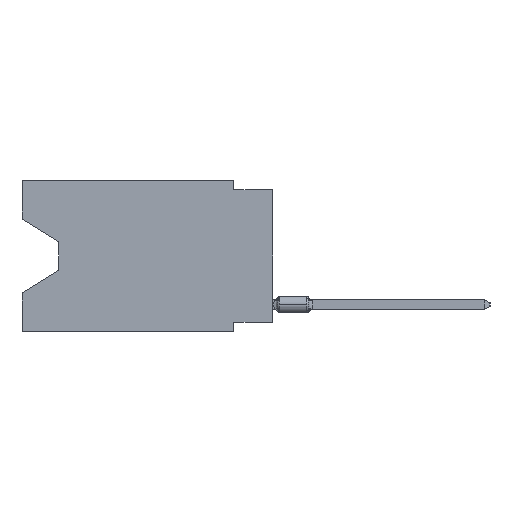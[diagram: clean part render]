
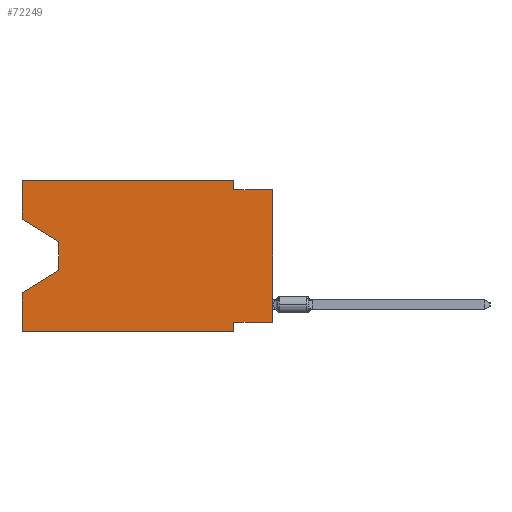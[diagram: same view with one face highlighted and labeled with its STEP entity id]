
A CAD part, left-side view. The second image highlights one B-rep face of the part: STEP entity #72249.
In plain terms, the highlighted planar face has unit normal (-1, 0, 0).
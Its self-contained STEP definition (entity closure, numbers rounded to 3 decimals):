
#250 = VECTOR ( 'NONE', #46614, 1000. ) ;
#735 = VERTEX_POINT ( 'NONE', #49858 ) ;
#942 = LINE ( 'NONE', #41583, #51331 ) ;
#1957 = VECTOR ( 'NONE', #62663, 1000. ) ;
#2201 = VECTOR ( 'NONE', #43357, 1000. ) ;
#4499 = ORIENTED_EDGE ( 'NONE', *, *, #11922, .T. ) ;
#5413 = LINE ( 'NONE', #52946, #5985 ) ;
#5985 = VECTOR ( 'NONE', #11177, 1000. ) ;
#7062 = DIRECTION ( 'NONE',  ( 0., -1., 0. ) ) ;
#7840 = DIRECTION ( 'NONE',  ( 0., 0., -1. ) ) ;
#7853 = VECTOR ( 'NONE', #40962, 1000. ) ;
#9256 = ORIENTED_EDGE ( 'NONE', *, *, #23784, .T. ) ;
#11087 = CARTESIAN_POINT ( 'NONE',  ( 0., 0., 0. ) ) ;
#11177 = DIRECTION ( 'NONE',  ( 0., 0., -1. ) ) ;
#11338 = CARTESIAN_POINT ( 'NONE',  ( 0., 16.383, -9.906 ) ) ;
#11922 = EDGE_CURVE ( 'NONE', #42010, #60804, #32183, .T. ) ;
#12858 = CARTESIAN_POINT ( 'NONE',  ( 0., 13.97, -5.893 ) ) ;
#14801 = VERTEX_POINT ( 'NONE', #21373 ) ;
#15666 = DIRECTION ( 'NONE',  ( 0., 0., -1. ) ) ;
#16259 = ORIENTED_EDGE ( 'NONE', *, *, #63961, .F. ) ;
#16802 = CARTESIAN_POINT ( 'NONE',  ( 0., 16.383, 0. ) ) ;
#17187 = PLANE ( 'NONE',  #37802 ) ;
#17555 = DIRECTION ( 'NONE',  ( 0., -1., 0. ) ) ;
#17570 = CARTESIAN_POINT ( 'NONE',  ( 0., 16.383, -2.546 ) ) ;
#17581 = DIRECTION ( 'NONE',  ( 0., 0., 1. ) ) ;
#18589 = LINE ( 'NONE', #58868, #64300 ) ;
#19601 = EDGE_CURVE ( 'NONE', #14801, #23653, #23713, .T. ) ;
#19914 = VERTEX_POINT ( 'NONE', #28621 ) ;
#21373 = CARTESIAN_POINT ( 'NONE',  ( 0., 0., -9.271 ) ) ;
#21860 = ORIENTED_EDGE ( 'NONE', *, *, #73483, .F. ) ;
#22538 = VERTEX_POINT ( 'NONE', #23243 ) ;
#22686 = CARTESIAN_POINT ( 'NONE',  ( 0., 2.54, -9.906 ) ) ;
#23243 = CARTESIAN_POINT ( 'NONE',  ( 0., 2.54, -0.635 ) ) ;
#23653 = VERTEX_POINT ( 'NONE', #51052 ) ;
#23700 = LINE ( 'NONE', #17570, #7853 ) ;
#23713 = LINE ( 'NONE', #11087, #52061 ) ;
#23784 = EDGE_CURVE ( 'NONE', #53738, #42010, #5413, .T. ) ;
#27193 = CARTESIAN_POINT ( 'NONE',  ( 0., 13.97, -5.893 ) ) ;
#28321 = FACE_OUTER_BOUND ( 'NONE', #30038, .T. ) ;
#28621 = CARTESIAN_POINT ( 'NONE',  ( 0., 16.383, -9.906 ) ) ;
#29173 = EDGE_CURVE ( 'NONE', #72198, #735, #68787, .T. ) ;
#29593 = VERTEX_POINT ( 'NONE', #22686 ) ;
#30038 = EDGE_LOOP ( 'NONE', ( #52075, #9256, #4499, #45428, #39460, #21860, #72965, #66059, #16259, #39296, #55247, #48115 ) ) ;
#30872 = CARTESIAN_POINT ( 'NONE',  ( 0., 2.54, 0. ) ) ;
#32183 = LINE ( 'NONE', #27193, #49501 ) ;
#33424 = VERTEX_POINT ( 'NONE', #30872 ) ;
#37661 = CARTESIAN_POINT ( 'NONE',  ( 0., 0., -9.271 ) ) ;
#37802 = AXIS2_PLACEMENT_3D ( 'NONE', #16802, #63589, #15666 ) ;
#38332 = CARTESIAN_POINT ( 'NONE',  ( 0., 16.383, 0. ) ) ;
#39296 = ORIENTED_EDGE ( 'NONE', *, *, #40790, .F. ) ;
#39309 = EDGE_CURVE ( 'NONE', #19914, #29593, #58099, .T. ) ;
#39460 = ORIENTED_EDGE ( 'NONE', *, *, #39309, .T. ) ;
#40046 = VECTOR ( 'NONE', #72459, 1000. ) ;
#40299 = CARTESIAN_POINT ( 'NONE',  ( 0., 13.97, -4.013 ) ) ;
#40790 = EDGE_CURVE ( 'NONE', #33424, #22538, #18589, .T. ) ;
#40962 = DIRECTION ( 'NONE',  ( 0., -0.855, -0.519 ) ) ;
#41583 = CARTESIAN_POINT ( 'NONE',  ( 0., 0., -0.635 ) ) ;
#42010 = VERTEX_POINT ( 'NONE', #12858 ) ;
#43023 = LINE ( 'NONE', #37661, #58078 ) ;
#43357 = DIRECTION ( 'NONE',  ( 0., 0., -1. ) ) ;
#43681 = DIRECTION ( 'NONE',  ( 0., 0.855, -0.519 ) ) ;
#44074 = EDGE_CURVE ( 'NONE', #19914, #60804, #54825, .T. ) ;
#44807 = CARTESIAN_POINT ( 'NONE',  ( 0., 16.383, -2.546 ) ) ;
#45428 = ORIENTED_EDGE ( 'NONE', *, *, #44074, .F. ) ;
#46614 = DIRECTION ( 'NONE',  ( 0., -1., 0. ) ) ;
#48115 = ORIENTED_EDGE ( 'NONE', *, *, #29173, .F. ) ;
#49501 = VECTOR ( 'NONE', #43681, 1000. ) ;
#49858 = CARTESIAN_POINT ( 'NONE',  ( 0., 16.383, 0. ) ) ;
#51052 = CARTESIAN_POINT ( 'NONE',  ( 0., 0., -0.635 ) ) ;
#51331 = VECTOR ( 'NONE', #7062, 1000. ) ;
#52061 = VECTOR ( 'NONE', #17581, 1000. ) ;
#52075 = ORIENTED_EDGE ( 'NONE', *, *, #67397, .T. ) ;
#52946 = CARTESIAN_POINT ( 'NONE',  ( 0., 13.97, -4.013 ) ) ;
#53738 = VERTEX_POINT ( 'NONE', #40299 ) ;
#54825 = LINE ( 'NONE', #38332, #40046 ) ;
#55247 = ORIENTED_EDGE ( 'NONE', *, *, #55536, .F. ) ;
#55536 = EDGE_CURVE ( 'NONE', #735, #33424, #63582, .T. ) ;
#55588 = CARTESIAN_POINT ( 'NONE',  ( 0., 16.383, -7.36 ) ) ;
#56597 = EDGE_CURVE ( 'NONE', #14801, #69345, #43023, .T. ) ;
#58039 = CARTESIAN_POINT ( 'NONE',  ( 0., 16.383, 0. ) ) ;
#58078 = VECTOR ( 'NONE', #61040, 1000. ) ;
#58099 = LINE ( 'NONE', #11338, #250 ) ;
#58195 = CARTESIAN_POINT ( 'NONE',  ( 0., 16.383, 0. ) ) ;
#58868 = CARTESIAN_POINT ( 'NONE',  ( 0., 2.54, 0. ) ) ;
#59872 = LINE ( 'NONE', #72493, #2201 ) ;
#60804 = VERTEX_POINT ( 'NONE', #55588 ) ;
#61040 = DIRECTION ( 'NONE',  ( 0., 1., 0. ) ) ;
#62663 = DIRECTION ( 'NONE',  ( 0., 0., 1. ) ) ;
#63582 = LINE ( 'NONE', #58195, #66591 ) ;
#63589 = DIRECTION ( 'NONE',  ( 1., 0., 0. ) ) ;
#63961 = EDGE_CURVE ( 'NONE', #22538, #23653, #942, .T. ) ;
#64300 = VECTOR ( 'NONE', #7840, 1000. ) ;
#64312 = CARTESIAN_POINT ( 'NONE',  ( 0., 2.54, -9.271 ) ) ;
#66059 = ORIENTED_EDGE ( 'NONE', *, *, #19601, .T. ) ;
#66591 = VECTOR ( 'NONE', #17555, 1000. ) ;
#67397 = EDGE_CURVE ( 'NONE', #72198, #53738, #23700, .T. ) ;
#68787 = LINE ( 'NONE', #58039, #1957 ) ;
#69345 = VERTEX_POINT ( 'NONE', #64312 ) ;
#72198 = VERTEX_POINT ( 'NONE', #44807 ) ;
#72249 = ADVANCED_FACE ( 'NONE', ( #28321 ), #17187, .F. ) ;
#72459 = DIRECTION ( 'NONE',  ( 0., 0., 1. ) ) ;
#72493 = CARTESIAN_POINT ( 'NONE',  ( 0., 2.54, -9.906 ) ) ;
#72965 = ORIENTED_EDGE ( 'NONE', *, *, #56597, .F. ) ;
#73483 = EDGE_CURVE ( 'NONE', #69345, #29593, #59872, .T. ) ;
